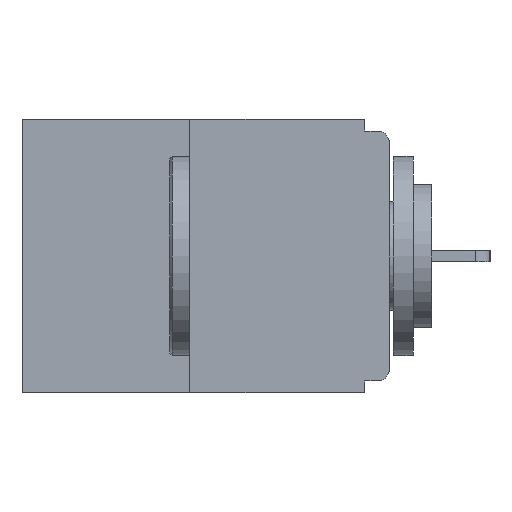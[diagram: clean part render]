
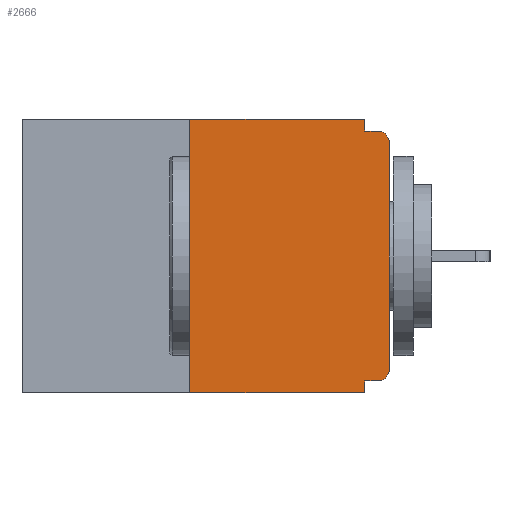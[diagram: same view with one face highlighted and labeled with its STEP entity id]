
A CAD part, left-side view. The second image highlights one B-rep face of the part: STEP entity #2666.
In plain terms, the highlighted planar face has unit normal (-1, 0, 0).
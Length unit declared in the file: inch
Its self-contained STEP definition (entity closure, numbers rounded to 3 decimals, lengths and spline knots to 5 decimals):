
#18 = CARTESIAN_POINT ( 'NONE',  ( 0., 0.25, 0. ) ) ;
#232 = DIRECTION ( 'NONE',  ( 0., 0., -1. ) ) ;
#490 = VERTEX_POINT ( 'NONE', #10916 ) ;
#533 = ORIENTED_EDGE ( 'NONE', *, *, #5032, .T. ) ;
#951 = CARTESIAN_POINT ( 'NONE',  ( 0., 0.46, 0. ) ) ;
#991 = VECTOR ( 'NONE', #5641, 39.37008 ) ;
#1050 = EDGE_CURVE ( 'NONE', #4587, #9281, #8802, .T. ) ;
#1203 = VERTEX_POINT ( 'NONE', #7248 ) ;
#1227 = ORIENTED_EDGE ( 'NONE', *, *, #8661, .T. ) ;
#1367 = CARTESIAN_POINT ( 'NONE',  ( 0., 0., 0. ) ) ;
#1796 = CIRCLE ( 'NONE', #2841, 0.015 ) ;
#1868 = VECTOR ( 'NONE', #10203, 39.37008 ) ;
#1878 = VERTEX_POINT ( 'NONE', #11687 ) ;
#1888 = LINE ( 'NONE', #951, #1996 ) ;
#1931 = ORIENTED_EDGE ( 'NONE', *, *, #11782, .F. ) ;
#1996 = VECTOR ( 'NONE', #6014, 39.37008 ) ;
#2031 = DIRECTION ( 'NONE',  ( 0., 1., 0. ) ) ;
#2148 = DIRECTION ( 'NONE',  ( -1., 0., 0. ) ) ;
#2155 = ORIENTED_EDGE ( 'NONE', *, *, #11681, .F. ) ;
#2212 = CARTESIAN_POINT ( 'NONE',  ( 0., 0.015, -0.03 ) ) ;
#2281 = DIRECTION ( 'NONE',  ( 0., -1., 0. ) ) ;
#2314 = ORIENTED_EDGE ( 'NONE', *, *, #8662, .F. ) ;
#2364 = LINE ( 'NONE', #1367, #12636 ) ;
#2381 = LINE ( 'NONE', #6371, #1868 ) ;
#2487 = CARTESIAN_POINT ( 'NONE',  ( 0., 0.031, 0. ) ) ;
#2655 = VERTEX_POINT ( 'NONE', #9918 ) ;
#2666 = ADVANCED_FACE ( 'NONE', ( #8991 ), #10054, .F. ) ;
#2763 = EDGE_CURVE ( 'NONE', #11255, #9363, #4188, .T. ) ;
#2841 = AXIS2_PLACEMENT_3D ( 'NONE', #2212, #2148, #232 ) ;
#2983 = ORIENTED_EDGE ( 'NONE', *, *, #2763, .F. ) ;
#3177 = VERTEX_POINT ( 'NONE', #5943 ) ;
#3184 = LINE ( 'NONE', #11184, #6396 ) ;
#3197 = DIRECTION ( 'NONE',  ( 0., 0., -1. ) ) ;
#3403 = ORIENTED_EDGE ( 'NONE', *, *, #11892, .T. ) ;
#3465 = DIRECTION ( 'NONE',  ( 0., 0., -1. ) ) ;
#4188 = LINE ( 'NONE', #5173, #6153 ) ;
#4446 = EDGE_LOOP ( 'NONE', ( #1931, #5131, #533, #2314, #2983, #11986, #1227, #3403, #9462, #2155 ) ) ;
#4583 = CIRCLE ( 'NONE', #7713, 0.015 ) ;
#4587 = VERTEX_POINT ( 'NONE', #7183 ) ;
#4683 = AXIS2_PLACEMENT_3D ( 'NONE', #10177, #9181, #3197 ) ;
#4706 = VECTOR ( 'NONE', #5749, 39.37008 ) ;
#5032 = EDGE_CURVE ( 'NONE', #4587, #490, #3184, .T. ) ;
#5103 = CARTESIAN_POINT ( 'NONE',  ( 0., 0.031, 0. ) ) ;
#5131 = ORIENTED_EDGE ( 'NONE', *, *, #1050, .F. ) ;
#5173 = CARTESIAN_POINT ( 'NONE',  ( 0., 0., -0.328 ) ) ;
#5558 = LINE ( 'NONE', #2487, #4706 ) ;
#5641 = DIRECTION ( 'NONE',  ( 0., 0., 1. ) ) ;
#5749 = DIRECTION ( 'NONE',  ( 0., 0., -1. ) ) ;
#5877 = DIRECTION ( 'NONE',  ( 0., 0., 1. ) ) ;
#5943 = CARTESIAN_POINT ( 'NONE',  ( 0., 0.015, -0.015 ) ) ;
#6014 = DIRECTION ( 'NONE',  ( 0., -1., 0. ) ) ;
#6153 = VECTOR ( 'NONE', #2031, 39.37008 ) ;
#6371 = CARTESIAN_POINT ( 'NONE',  ( 0., 0., -0.015 ) ) ;
#6396 = VECTOR ( 'NONE', #2281, 39.37008 ) ;
#7183 = CARTESIAN_POINT ( 'NONE',  ( 0., 0.25, -0.343 ) ) ;
#7248 = CARTESIAN_POINT ( 'NONE',  ( 0., 0., -0.03 ) ) ;
#7713 = AXIS2_PLACEMENT_3D ( 'NONE', #7791, #8510, #10524 ) ;
#7791 = CARTESIAN_POINT ( 'NONE',  ( 0., 0.015, -0.313 ) ) ;
#8510 = DIRECTION ( 'NONE',  ( -1., 0., 0. ) ) ;
#8661 = EDGE_CURVE ( 'NONE', #1878, #1203, #2364, .T. ) ;
#8662 = EDGE_CURVE ( 'NONE', #9363, #490, #8786, .T. ) ;
#8786 = LINE ( 'NONE', #9529, #10330 ) ;
#8802 = LINE ( 'NONE', #10700, #991 ) ;
#8991 = FACE_OUTER_BOUND ( 'NONE', #4446, .T. ) ;
#9181 = DIRECTION ( 'NONE',  ( 1., 0., 0. ) ) ;
#9281 = VERTEX_POINT ( 'NONE', #18 ) ;
#9363 = VERTEX_POINT ( 'NONE', #11100 ) ;
#9462 = ORIENTED_EDGE ( 'NONE', *, *, #9485, .F. ) ;
#9485 = EDGE_CURVE ( 'NONE', #2655, #3177, #2381, .T. ) ;
#9529 = CARTESIAN_POINT ( 'NONE',  ( 0., 0.031, -0.343 ) ) ;
#9610 = EDGE_CURVE ( 'NONE', #11255, #1878, #4583, .T. ) ;
#9918 = CARTESIAN_POINT ( 'NONE',  ( 0., 0.031, -0.015 ) ) ;
#10054 = PLANE ( 'NONE',  #4683 ) ;
#10177 = CARTESIAN_POINT ( 'NONE',  ( 0., 0.46, 0. ) ) ;
#10203 = DIRECTION ( 'NONE',  ( 0., -1., 0. ) ) ;
#10330 = VECTOR ( 'NONE', #3465, 39.37008 ) ;
#10524 = DIRECTION ( 'NONE',  ( 0., 0., -1. ) ) ;
#10700 = CARTESIAN_POINT ( 'NONE',  ( 0., 0.25, 0. ) ) ;
#10916 = CARTESIAN_POINT ( 'NONE',  ( 0., 0.031, -0.343 ) ) ;
#11100 = CARTESIAN_POINT ( 'NONE',  ( 0., 0.031, -0.328 ) ) ;
#11184 = CARTESIAN_POINT ( 'NONE',  ( 0., 0.46, -0.343 ) ) ;
#11255 = VERTEX_POINT ( 'NONE', #11623 ) ;
#11436 = VERTEX_POINT ( 'NONE', #5103 ) ;
#11623 = CARTESIAN_POINT ( 'NONE',  ( 0., 0.015, -0.328 ) ) ;
#11681 = EDGE_CURVE ( 'NONE', #11436, #2655, #5558, .T. ) ;
#11687 = CARTESIAN_POINT ( 'NONE',  ( 0., 0., -0.313 ) ) ;
#11782 = EDGE_CURVE ( 'NONE', #9281, #11436, #1888, .T. ) ;
#11892 = EDGE_CURVE ( 'NONE', #1203, #3177, #1796, .T. ) ;
#11986 = ORIENTED_EDGE ( 'NONE', *, *, #9610, .T. ) ;
#12636 = VECTOR ( 'NONE', #5877, 39.37008 ) ;
